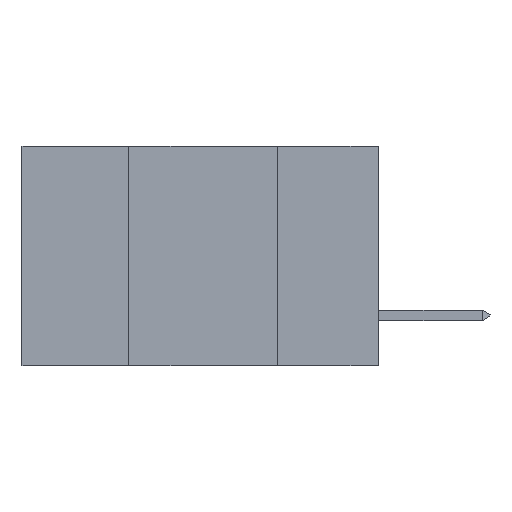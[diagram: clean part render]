
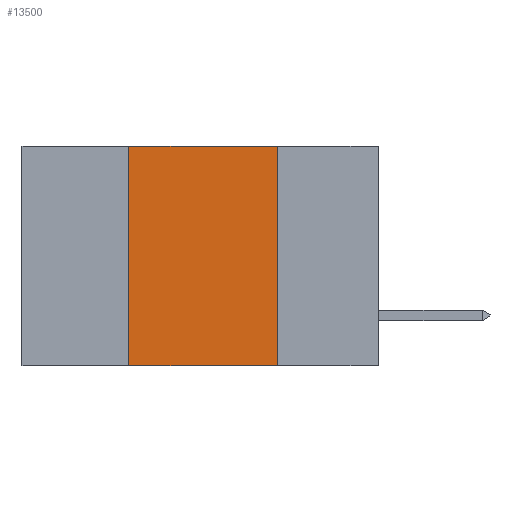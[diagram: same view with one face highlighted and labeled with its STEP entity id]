
A CAD part, left-side view. The second image highlights one B-rep face of the part: STEP entity #13500.
In plain terms, the highlighted planar face has unit normal (-1, 0, 0).
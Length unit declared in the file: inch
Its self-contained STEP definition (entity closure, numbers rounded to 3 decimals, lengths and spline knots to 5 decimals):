
#1872 = LINE ( 'NONE', #13335, #18510 ) ;
#2079 = ORIENTED_EDGE ( 'NONE', *, *, #23251, .F. ) ;
#2851 = CARTESIAN_POINT ( 'NONE',  ( 0., 0.17, -0.37 ) ) ;
#2869 = EDGE_CURVE ( 'NONE', #7772, #20401, #7408, .T. ) ;
#3534 = CARTESIAN_POINT ( 'NONE',  ( 0., 0.6, -0.37 ) ) ;
#4021 = FACE_OUTER_BOUND ( 'NONE', #24627, .T. ) ;
#4328 = VECTOR ( 'NONE', #23489, 39.37008 ) ;
#4788 = EDGE_CURVE ( 'NONE', #17097, #16572, #20933, .T. ) ;
#5297 = AXIS2_PLACEMENT_3D ( 'NONE', #6523, #12583, #15982 ) ;
#6523 = CARTESIAN_POINT ( 'NONE',  ( 0., 0.6, 0. ) ) ;
#7408 = LINE ( 'NONE', #3534, #4328 ) ;
#7772 = VERTEX_POINT ( 'NONE', #17117 ) ;
#8158 = ORIENTED_EDGE ( 'NONE', *, *, #15903, .F. ) ;
#8534 = PLANE ( 'NONE',  #5297 ) ;
#12583 = DIRECTION ( 'NONE',  ( 1., 0., 0. ) ) ;
#13287 = CARTESIAN_POINT ( 'NONE',  ( 0., 0.17, 0. ) ) ;
#13335 = CARTESIAN_POINT ( 'NONE',  ( 0., 0.17, -0.37 ) ) ;
#13500 = ADVANCED_FACE ( 'NONE', ( #4021 ), #8534, .F. ) ;
#14619 = DIRECTION ( 'NONE',  ( 0., 0., 1. ) ) ;
#14885 = CARTESIAN_POINT ( 'NONE',  ( 0., 0.42, 0. ) ) ;
#15136 = CARTESIAN_POINT ( 'NONE',  ( 0., 0.42, -0.37 ) ) ;
#15157 = VECTOR ( 'NONE', #25017, 39.37008 ) ;
#15903 = EDGE_CURVE ( 'NONE', #7772, #17097, #18566, .T. ) ;
#15982 = DIRECTION ( 'NONE',  ( 0., 0., -1. ) ) ;
#16572 = VERTEX_POINT ( 'NONE', #13287 ) ;
#16608 = ORIENTED_EDGE ( 'NONE', *, *, #4788, .F. ) ;
#17012 = CARTESIAN_POINT ( 'NONE',  ( 0., 0.6, 0. ) ) ;
#17097 = VERTEX_POINT ( 'NONE', #14885 ) ;
#17117 = CARTESIAN_POINT ( 'NONE',  ( 0., 0.42, -0.37 ) ) ;
#18510 = VECTOR ( 'NONE', #19482, 39.37008 ) ;
#18566 = LINE ( 'NONE', #15136, #22500 ) ;
#19482 = DIRECTION ( 'NONE',  ( 0., 0., -1. ) ) ;
#20401 = VERTEX_POINT ( 'NONE', #2851 ) ;
#20933 = LINE ( 'NONE', #17012, #15157 ) ;
#21546 = ORIENTED_EDGE ( 'NONE', *, *, #2869, .T. ) ;
#22500 = VECTOR ( 'NONE', #14619, 39.37008 ) ;
#23251 = EDGE_CURVE ( 'NONE', #16572, #20401, #1872, .T. ) ;
#23489 = DIRECTION ( 'NONE',  ( 0., -1., 0. ) ) ;
#24627 = EDGE_LOOP ( 'NONE', ( #2079, #16608, #8158, #21546 ) ) ;
#25017 = DIRECTION ( 'NONE',  ( 0., -1., 0. ) ) ;
